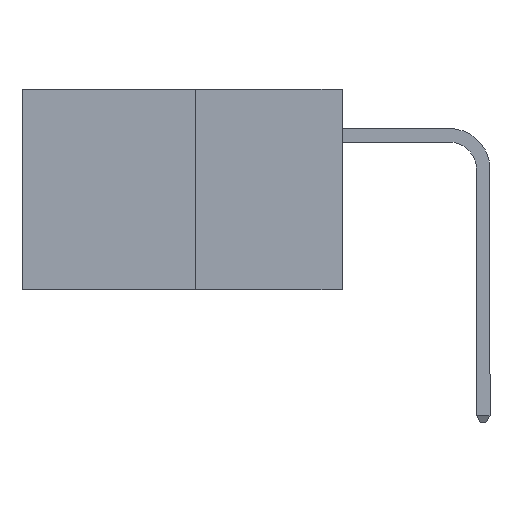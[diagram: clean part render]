
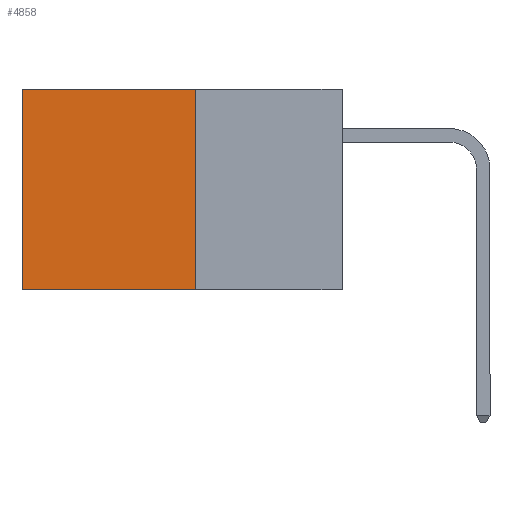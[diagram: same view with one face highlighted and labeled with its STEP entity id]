
A CAD part, left-side view. The second image highlights one B-rep face of the part: STEP entity #4858.
In plain terms, the highlighted planar face has unit normal (-1, 0, 0).
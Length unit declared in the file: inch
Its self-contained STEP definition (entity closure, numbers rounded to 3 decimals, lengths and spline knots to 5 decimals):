
#63 = DIRECTION ( 'NONE',  ( 0., 0., -1. ) ) ;
#75 = CARTESIAN_POINT ( 'NONE',  ( 0.277, 0.27, -0.37 ) ) ;
#166 = CARTESIAN_POINT ( 'NONE',  ( 0.277, 0.27, -0.37 ) ) ;
#804 = CARTESIAN_POINT ( 'NONE',  ( 0.277, 0.59, 0. ) ) ;
#815 = DIRECTION ( 'NONE',  ( 0., 1., 0. ) ) ;
#958 = CARTESIAN_POINT ( 'NONE',  ( 0.277, 0.59, -0.37 ) ) ;
#2558 = CARTESIAN_POINT ( 'NONE',  ( 0.277, 0.27, -0.37 ) ) ;
#2594 = DIRECTION ( 'NONE',  ( 0., 1., 0. ) ) ;
#2885 = EDGE_LOOP ( 'NONE', ( #3200, #3405, #6740, #7082 ) ) ;
#2916 = CARTESIAN_POINT ( 'NONE',  ( 0.277, 0.27, -0.37 ) ) ;
#2949 = EDGE_CURVE ( 'NONE', #4214, #4042, #6127, .T. ) ;
#2997 = DIRECTION ( 'NONE',  ( 0., 0., -1. ) ) ;
#3068 = DIRECTION ( 'NONE',  ( 1., 0., 0. ) ) ;
#3138 = CARTESIAN_POINT ( 'NONE',  ( 0.277, 0.59, -0.37 ) ) ;
#3200 = ORIENTED_EDGE ( 'NONE', *, *, #6188, .T. ) ;
#3228 = LINE ( 'NONE', #6073, #4680 ) ;
#3396 = AXIS2_PLACEMENT_3D ( 'NONE', #2558, #3068, #2997 ) ;
#3405 = ORIENTED_EDGE ( 'NONE', *, *, #4799, .F. ) ;
#3454 = VECTOR ( 'NONE', #4974, 39.37008 ) ;
#3481 = FACE_OUTER_BOUND ( 'NONE', #2885, .T. ) ;
#3633 = EDGE_CURVE ( 'NONE', #4214, #5284, #3228, .T. ) ;
#3674 = PLANE ( 'NONE',  #3396 ) ;
#3676 = VECTOR ( 'NONE', #2594, 39.37008 ) ;
#4042 = VERTEX_POINT ( 'NONE', #166 ) ;
#4047 = VERTEX_POINT ( 'NONE', #958 ) ;
#4214 = VERTEX_POINT ( 'NONE', #5418 ) ;
#4680 = VECTOR ( 'NONE', #815, 39.37008 ) ;
#4799 = EDGE_CURVE ( 'NONE', #4042, #4047, #6814, .T. ) ;
#4858 = ADVANCED_FACE ( 'NONE', ( #3481 ), #3674, .F. ) ;
#4974 = DIRECTION ( 'NONE',  ( 0., 0., -1. ) ) ;
#5056 = LINE ( 'NONE', #3138, #3454 ) ;
#5284 = VERTEX_POINT ( 'NONE', #804 ) ;
#5418 = CARTESIAN_POINT ( 'NONE',  ( 0.277, 0.27, 0. ) ) ;
#5933 = VECTOR ( 'NONE', #63, 39.37008 ) ;
#6073 = CARTESIAN_POINT ( 'NONE',  ( 0.277, 0.27, 0. ) ) ;
#6127 = LINE ( 'NONE', #75, #5933 ) ;
#6188 = EDGE_CURVE ( 'NONE', #5284, #4047, #5056, .T. ) ;
#6740 = ORIENTED_EDGE ( 'NONE', *, *, #2949, .F. ) ;
#6814 = LINE ( 'NONE', #2916, #3676 ) ;
#7082 = ORIENTED_EDGE ( 'NONE', *, *, #3633, .T. ) ;
